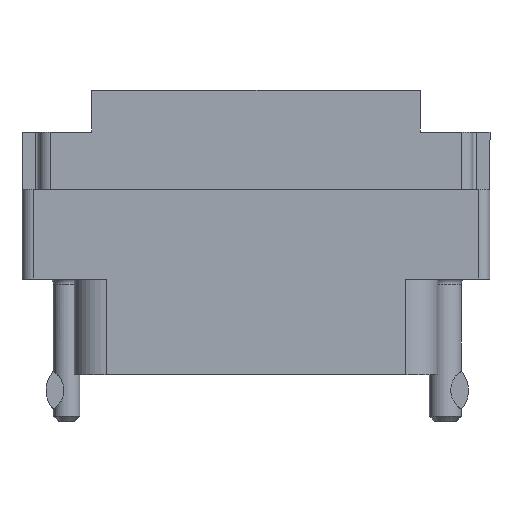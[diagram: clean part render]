
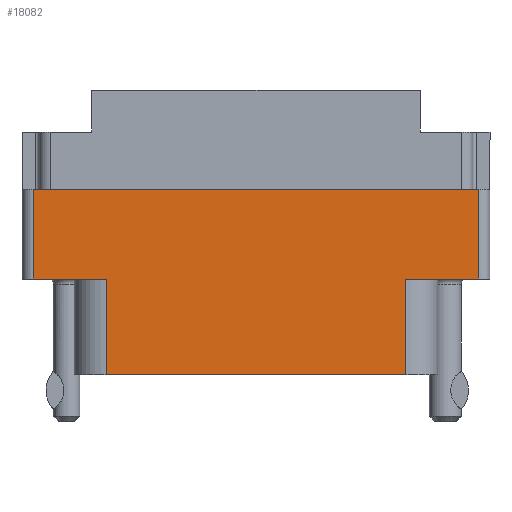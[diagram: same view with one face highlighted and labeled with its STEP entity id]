
A CAD part, front view. The second image highlights one B-rep face of the part: STEP entity #18082.
In plain terms, the highlighted planar face has unit normal (0, -1, 0).
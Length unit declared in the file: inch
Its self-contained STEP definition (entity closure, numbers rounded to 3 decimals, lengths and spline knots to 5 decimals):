
#148 = DIRECTION ( 'NONE',  ( 0., 0., 1. ) ) ;
#718 = CARTESIAN_POINT ( 'NONE',  ( 0., -0.343, -0.529 ) ) ;
#1012 = LINE ( 'NONE', #11544, #13461 ) ;
#1068 = ORIENTED_EDGE ( 'NONE', *, *, #1318, .F. ) ;
#1318 = EDGE_CURVE ( 'NONE', #10722, #27566, #1012, .T. ) ;
#1481 = ORIENTED_EDGE ( 'NONE', *, *, #17937, .F. ) ;
#1859 = CARTESIAN_POINT ( 'NONE',  ( -0.624, -0.343, -0.277 ) ) ;
#3244 = VECTOR ( 'NONE', #148, 39.37008 ) ;
#3487 = AXIS2_PLACEMENT_3D ( 'NONE', #20386, #13608, #8786 ) ;
#3872 = CARTESIAN_POINT ( 'NONE',  ( 0., -0.343, -0.529 ) ) ;
#3993 = VECTOR ( 'NONE', #5439, 39.37008 ) ;
#4094 = CARTESIAN_POINT ( 'NONE',  ( -0.624, -0.343, -0.798 ) ) ;
#4474 = CARTESIAN_POINT ( 'NONE',  ( 0.42, -0.343, -0.529 ) ) ;
#4703 = LINE ( 'NONE', #21070, #3244 ) ;
#5439 = DIRECTION ( 'NONE',  ( 1., 0., 0. ) ) ;
#5768 = LINE ( 'NONE', #4094, #14214 ) ;
#6631 = DIRECTION ( 'NONE',  ( 0., 0., 1. ) ) ;
#6767 = VECTOR ( 'NONE', #7482, 39.37008 ) ;
#7167 = LINE ( 'NONE', #19967, #9367 ) ;
#7270 = VERTEX_POINT ( 'NONE', #17258 ) ;
#7366 = LINE ( 'NONE', #7375, #17636 ) ;
#7375 = CARTESIAN_POINT ( 'NONE',  ( 0.42, -0.343, -0.529 ) ) ;
#7482 = DIRECTION ( 'NONE',  ( 0., 0., -1. ) ) ;
#8561 = ORIENTED_EDGE ( 'NONE', *, *, #13116, .T. ) ;
#8643 = LINE ( 'NONE', #3872, #11597 ) ;
#8786 = DIRECTION ( 'NONE',  ( 0., 0., -1. ) ) ;
#9229 = EDGE_LOOP ( 'NONE', ( #12037, #16211, #10680, #23944, #8561, #1481, #1068, #12916 ) ) ;
#9367 = VECTOR ( 'NONE', #29171, 39.37008 ) ;
#9528 = DIRECTION ( 'NONE',  ( 0., 0., -1. ) ) ;
#9936 = CARTESIAN_POINT ( 'NONE',  ( -0.42, -0.343, -0.529 ) ) ;
#10680 = ORIENTED_EDGE ( 'NONE', *, *, #20789, .F. ) ;
#10722 = VERTEX_POINT ( 'NONE', #23387 ) ;
#11544 = CARTESIAN_POINT ( 'NONE',  ( -0.624, -0.343, -0.798 ) ) ;
#11597 = VECTOR ( 'NONE', #15535, 39.37008 ) ;
#12037 = ORIENTED_EDGE ( 'NONE', *, *, #16419, .T. ) ;
#12613 = CARTESIAN_POINT ( 'NONE',  ( -0.42, -0.343, -0.798 ) ) ;
#12916 = ORIENTED_EDGE ( 'NONE', *, *, #24311, .T. ) ;
#13018 = FACE_OUTER_BOUND ( 'NONE', #9229, .T. ) ;
#13116 = EDGE_CURVE ( 'NONE', #7270, #26915, #4703, .T. ) ;
#13461 = VECTOR ( 'NONE', #6631, 39.37008 ) ;
#13560 = CARTESIAN_POINT ( 'NONE',  ( 0.42, -0.343, -0.798 ) ) ;
#13608 = DIRECTION ( 'NONE',  ( 0., -1., 0. ) ) ;
#14214 = VECTOR ( 'NONE', #20057, 39.37008 ) ;
#14703 = CARTESIAN_POINT ( 'NONE',  ( -0.42, -0.343, -0.529 ) ) ;
#15535 = DIRECTION ( 'NONE',  ( -1., 0., 0. ) ) ;
#16211 = ORIENTED_EDGE ( 'NONE', *, *, #27856, .T. ) ;
#16419 = EDGE_CURVE ( 'NONE', #30087, #27854, #23632, .T. ) ;
#16452 = LINE ( 'NONE', #718, #3993 ) ;
#17258 = CARTESIAN_POINT ( 'NONE',  ( 0.624, -0.343, -0.529 ) ) ;
#17636 = VECTOR ( 'NONE', #9528, 39.37008 ) ;
#17937 = EDGE_CURVE ( 'NONE', #27566, #26915, #7167, .T. ) ;
#18082 = ADVANCED_FACE ( 'NONE', ( #13018 ), #25456, .T. ) ;
#18687 = CARTESIAN_POINT ( 'NONE',  ( 0.624, -0.343, -0.277 ) ) ;
#19967 = CARTESIAN_POINT ( 'NONE',  ( -0.656, -0.343, -0.277 ) ) ;
#20057 = DIRECTION ( 'NONE',  ( 1., 0., 0. ) ) ;
#20386 = CARTESIAN_POINT ( 'NONE',  ( -0.624, -0.343, -0.798 ) ) ;
#20789 = EDGE_CURVE ( 'NONE', #21755, #26887, #7366, .T. ) ;
#21070 = CARTESIAN_POINT ( 'NONE',  ( 0.624, -0.343, -0.798 ) ) ;
#21755 = VERTEX_POINT ( 'NONE', #4474 ) ;
#23387 = CARTESIAN_POINT ( 'NONE',  ( -0.624, -0.343, -0.529 ) ) ;
#23632 = LINE ( 'NONE', #9936, #6767 ) ;
#23944 = ORIENTED_EDGE ( 'NONE', *, *, #29710, .F. ) ;
#24311 = EDGE_CURVE ( 'NONE', #10722, #30087, #16452, .T. ) ;
#25456 = PLANE ( 'NONE',  #3487 ) ;
#26887 = VERTEX_POINT ( 'NONE', #13560 ) ;
#26915 = VERTEX_POINT ( 'NONE', #18687 ) ;
#27566 = VERTEX_POINT ( 'NONE', #1859 ) ;
#27854 = VERTEX_POINT ( 'NONE', #12613 ) ;
#27856 = EDGE_CURVE ( 'NONE', #27854, #26887, #5768, .T. ) ;
#29171 = DIRECTION ( 'NONE',  ( 1., 0., 0. ) ) ;
#29710 = EDGE_CURVE ( 'NONE', #7270, #21755, #8643, .T. ) ;
#30087 = VERTEX_POINT ( 'NONE', #14703 ) ;
